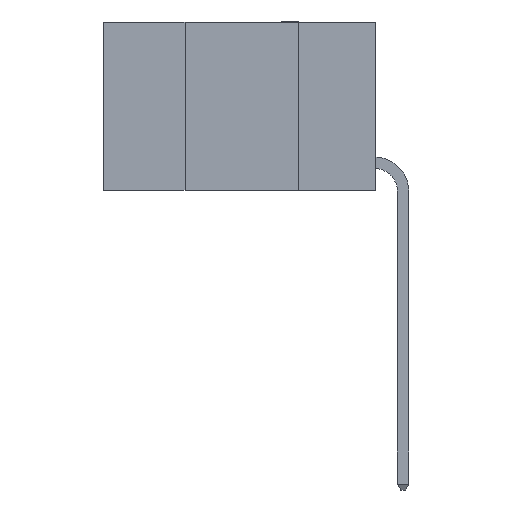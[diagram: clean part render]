
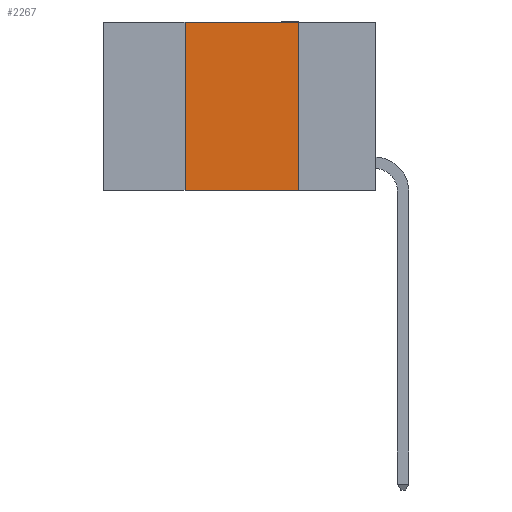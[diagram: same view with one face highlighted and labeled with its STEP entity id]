
A CAD part, left-side view. The second image highlights one B-rep face of the part: STEP entity #2267.
In plain terms, the highlighted planar face has unit normal (-1, 0, 0).
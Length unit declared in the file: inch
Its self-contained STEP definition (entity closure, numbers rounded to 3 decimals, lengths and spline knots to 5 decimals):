
#49 = VERTEX_POINT ( 'NONE', #5872 ) ;
#107 = CARTESIAN_POINT ( 'NONE',  ( 0., 0.42, 0. ) ) ;
#301 = EDGE_LOOP ( 'NONE', ( #7796, #4233, #2567, #6338 ) ) ;
#719 = VECTOR ( 'NONE', #5975, 39.37008 ) ;
#839 = CARTESIAN_POINT ( 'NONE',  ( 0., 0.42, 0. ) ) ;
#1424 = VECTOR ( 'NONE', #3231, 39.37008 ) ;
#1827 = VERTEX_POINT ( 'NONE', #107 ) ;
#1828 = AXIS2_PLACEMENT_3D ( 'NONE', #5126, #3749, #8716 ) ;
#2101 = LINE ( 'NONE', #2166, #9415 ) ;
#2166 = CARTESIAN_POINT ( 'NONE',  ( 0., 0.6, -0.37 ) ) ;
#2267 = ADVANCED_FACE ( 'NONE', ( #3734 ), #8007, .F. ) ;
#2372 = EDGE_CURVE ( 'NONE', #3565, #1827, #2621, .T. ) ;
#2567 = ORIENTED_EDGE ( 'NONE', *, *, #2372, .F. ) ;
#2621 = LINE ( 'NONE', #839, #719 ) ;
#3231 = DIRECTION ( 'NONE',  ( 0., 0., -1. ) ) ;
#3565 = VERTEX_POINT ( 'NONE', #5811 ) ;
#3734 = FACE_OUTER_BOUND ( 'NONE', #301, .T. ) ;
#3749 = DIRECTION ( 'NONE',  ( 1., 0., 0. ) ) ;
#4233 = ORIENTED_EDGE ( 'NONE', *, *, #8554, .F. ) ;
#4350 = VERTEX_POINT ( 'NONE', #8286 ) ;
#4581 = VECTOR ( 'NONE', #6512, 39.37008 ) ;
#4593 = EDGE_CURVE ( 'NONE', #3565, #49, #2101, .T. ) ;
#5126 = CARTESIAN_POINT ( 'NONE',  ( 0., 0.6, 0. ) ) ;
#5811 = CARTESIAN_POINT ( 'NONE',  ( 0., 0.42, -0.37 ) ) ;
#5872 = CARTESIAN_POINT ( 'NONE',  ( 0., 0.17, -0.37 ) ) ;
#5975 = DIRECTION ( 'NONE',  ( 0., 0., 1. ) ) ;
#6338 = ORIENTED_EDGE ( 'NONE', *, *, #4593, .T. ) ;
#6436 = DIRECTION ( 'NONE',  ( 0., -1., 0. ) ) ;
#6487 = LINE ( 'NONE', #7230, #4581 ) ;
#6512 = DIRECTION ( 'NONE',  ( 0., -1., 0. ) ) ;
#7210 = EDGE_CURVE ( 'NONE', #4350, #49, #8842, .T. ) ;
#7230 = CARTESIAN_POINT ( 'NONE',  ( 0., 0.6, 0. ) ) ;
#7796 = ORIENTED_EDGE ( 'NONE', *, *, #7210, .F. ) ;
#8007 = PLANE ( 'NONE',  #1828 ) ;
#8286 = CARTESIAN_POINT ( 'NONE',  ( 0., 0.17, 0. ) ) ;
#8554 = EDGE_CURVE ( 'NONE', #1827, #4350, #6487, .T. ) ;
#8716 = DIRECTION ( 'NONE',  ( 0., 0., -1. ) ) ;
#8842 = LINE ( 'NONE', #8888, #1424 ) ;
#8888 = CARTESIAN_POINT ( 'NONE',  ( 0., 0.17, 0. ) ) ;
#9415 = VECTOR ( 'NONE', #6436, 39.37008 ) ;
